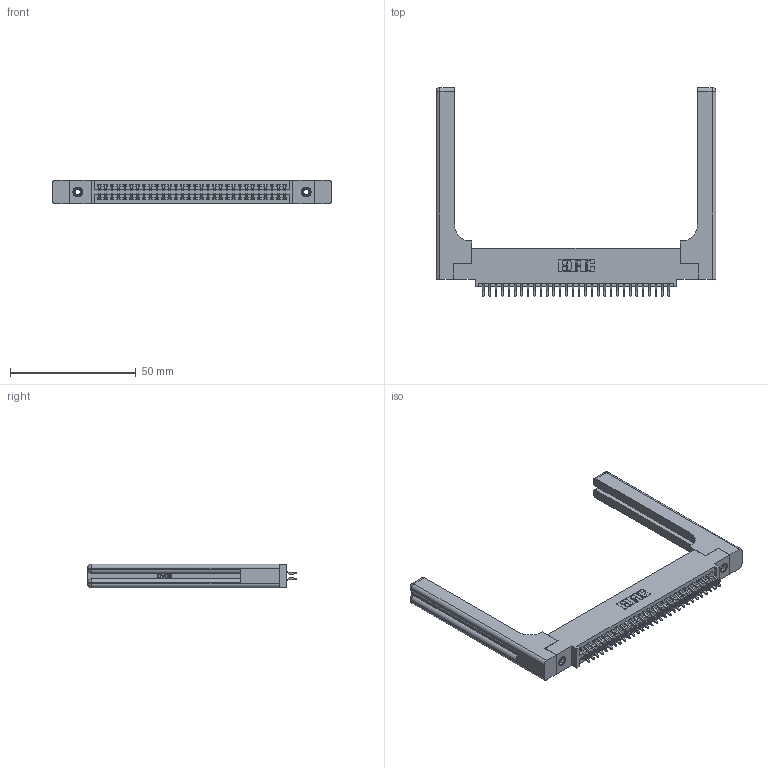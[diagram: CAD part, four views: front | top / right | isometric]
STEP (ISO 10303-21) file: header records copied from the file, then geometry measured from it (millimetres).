
FILE_DESCRIPTION (( 'STEP AP203' ), '1' );
FILE_NAME ('395-060-556-558.STEP', '2019-10-23T14:47:15', ( '' ), ( '' ), 'SwSTEP 2.0', 'SolidWorks 2016', '' );
FILE_SCHEMA (( 'CONFIG_CONTROL_DESIGN' ));
Length unit declared in the file: inch
Products named in the file (5): 345-250-001_345-250-001-102; 345-220-058_345-220-058; 345 Part_0.110 Offset - 0.156 Dia-TH; 395-060-556-558; 345-292-001_556 Tail
Assembly tree (65 placements, depth 2):
  395-060-556-558
    345 Part_0.110 Offset - 0.156 Dia-TH
    345-292-001_556 Tail  x60
    345-250-001_345-250-001-102  x2
    345-220-058_345-220-058  x2
Bounding box: 111.23 x 82.99 x 9.4 mm (x, y, z)
Volume: 19092.6 mm3; surface area: 20561.3 mm2
Topology: 65 solids, 65 shells, 3746 faces, 11039 edges, 7258 vertices
Faces by surface type: plane 2452, cylinder 1234, bspline 36, cone 12, sphere 8, torus 4
Entity records: 30688 total; most frequent: CARTESIAN_POINT 6165, ORIENTED_EDGE 4884, DIRECTION 4370, EDGE_CURVE 2442, VECTOR 2090, LINE 2090, VERTEX_POINT 1618, AXIS2_PLACEMENT_3D 1140
